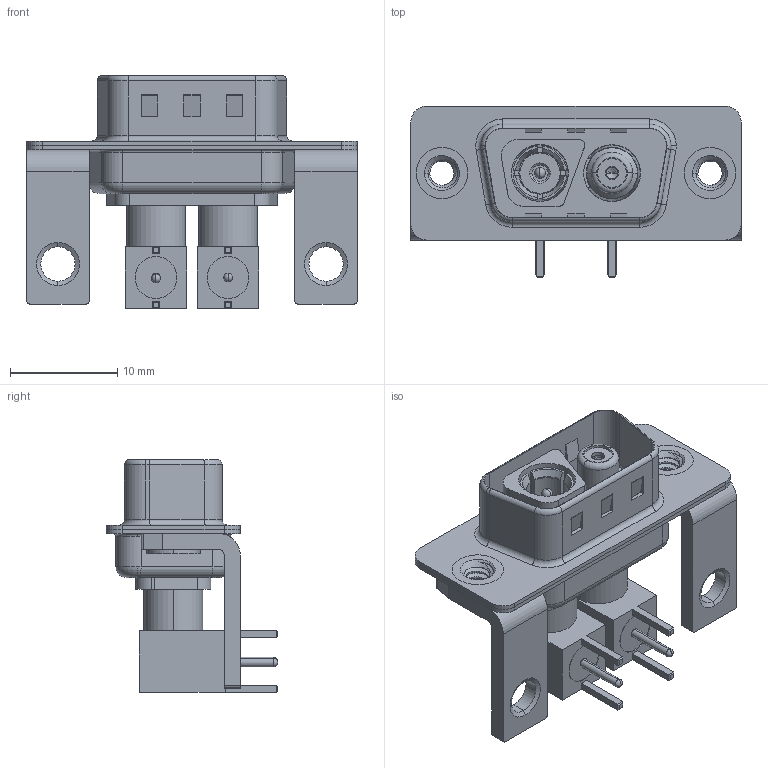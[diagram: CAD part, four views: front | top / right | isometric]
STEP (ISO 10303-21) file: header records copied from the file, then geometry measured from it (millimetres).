
FILE_DESCRIPTION (( 'STEP AP203' ), '1' );
FILE_NAME ('629-2WK2640-5N4.STEP', '2022-05-04T23:58:13', ( '' ), ( '' ), 'SwSTEP 2.0', 'SolidWorks 2020', '' );
FILE_SCHEMA (( 'CONFIG_CONTROL_DESIGN' ));
Length unit declared in the file: millimetre
Products named in the file (18): 629Combo Housing_2WK2; 629-2WK2640-5N4; Locking Collar; 629Combo Shell Rear_09 Contacts; RA Back Shell; Insulator Socket; Insulator RA Pin; Pin_RA; 629Combo Threaded Rivet_3; Socket_RA; 629Combo Stabilizer Bracket; Insulator Socket 2; Co-Ax Jack_RA PC Tail; Insulator Pin_Straight PC Tail; 629Combo Shell Front_09 Contacts; Co-Ax Jack Assy_RA; Co-Ax Plug_RA PC Tail; Co-Ax Plug Assy_RA
Assembly tree (22 placements, depth 3):
  629-2WK2640-5N4
    629Combo Housing_2WK2
    629Combo Shell Rear_09 Contacts
    629Combo Shell Front_09 Contacts
    629Combo Threaded Rivet_3  x2
    629Combo Stabilizer Bracket  x2
    Co-Ax Plug Assy_RA
      Co-Ax Plug_RA PC Tail
      Insulator Pin_Straight PC Tail
      Pin_RA
      Locking Collar
      RA Back Shell
      Insulator RA Pin
    Co-Ax Jack Assy_RA
      Co-Ax Jack_RA PC Tail
      Insulator Socket
      Insulator Socket 2
      Locking Collar
      Socket_RA
      RA Back Shell
      Insulator RA Pin
Bounding box: 30.8 x 16 x 21.71 mm (x, y, z)
Volume: 2260.9 mm3; surface area: 6186.2 mm2
Topology: 20 solids, 20 shells, 674 faces, 1636 edges, 1026 vertices
Faces by surface type: cylinder 284, plane 256, torus 62, cone 58, bspline 8, sphere 6
Entity records: 20186 total; most frequent: CARTESIAN_POINT 4543, DIRECTION 3057, ORIENTED_EDGE 2698, EDGE_CURVE 1349, AXIS2_PLACEMENT_3D 1196, VERTEX_POINT 854, VECTOR 665, LINE 665
